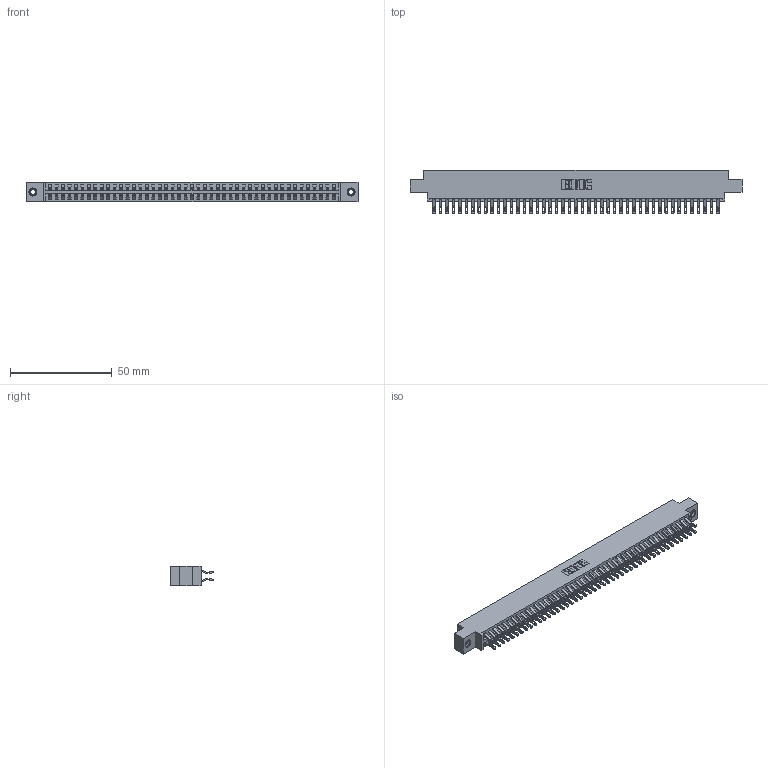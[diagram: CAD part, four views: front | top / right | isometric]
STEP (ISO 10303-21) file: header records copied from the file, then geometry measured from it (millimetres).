
FILE_DESCRIPTION (( 'STEP AP203' ), '1' );
FILE_NAME ('346-090-555-807.STEP', '2022-05-26T04:38:42', ( '' ), ( '' ), 'SwSTEP 2.0', 'SolidWorks 2020', '' );
FILE_SCHEMA (( 'CONFIG_CONTROL_DESIGN' ));
Length unit declared in the file: inch
Products named in the file (4): 346 Part_0.170 Offset - 0.156 Dia-TI; 345-250-001_345-250-005-103; 345-292-001_555 Tail; 346-090-555-807
Assembly tree (93 placements, depth 2):
  346-090-555-807
    346 Part_0.170 Offset - 0.156 Dia-TI
    345-292-001_555 Tail  x90
    345-250-001_345-250-005-103  x2
Bounding box: 163.45 x 21.46 x 9.4 mm (x, y, z)
Volume: 16054.5 mm3; surface area: 23259.1 mm2
Topology: 93 solids, 93 shells, 5406 faces, 16947 edges, 11290 vertices
Faces by surface type: plane 3082, cylinder 2308, cone 12, torus 4
Entity records: 30608 total; most frequent: CARTESIAN_POINT 5061, ORIENTED_EDGE 4958, DIRECTION 4505, EDGE_CURVE 2479, VECTOR 2127, LINE 2127, VERTEX_POINT 1648, AXIS2_PLACEMENT_3D 1189
